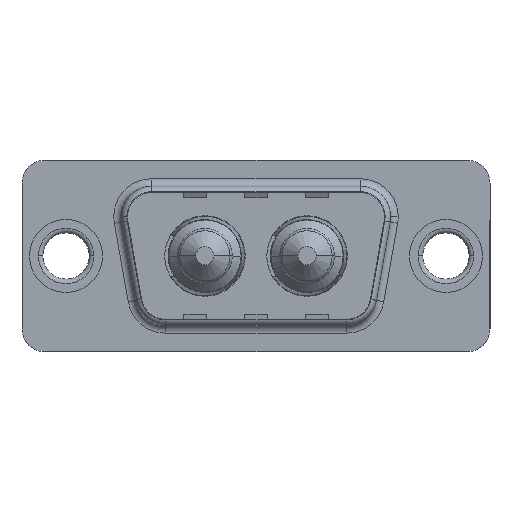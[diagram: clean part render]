
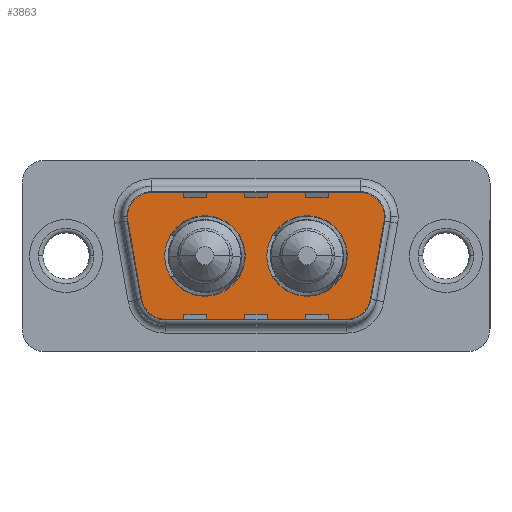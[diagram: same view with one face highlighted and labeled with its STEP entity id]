
A CAD part, top view. The second image highlights one B-rep face of the part: STEP entity #3863.
In plain terms, the highlighted planar face has unit normal (0, 0, 1).
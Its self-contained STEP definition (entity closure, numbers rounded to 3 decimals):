
#80 = VECTOR ( 'NONE', #3005, 1000. ) ;
#136 = CARTESIAN_POINT ( 'NONE',  ( 20.511, -3.247, 0. ) ) ;
#163 = EDGE_LOOP ( 'NONE', ( #2685, #4024 ) ) ;
#208 = VECTOR ( 'NONE', #8094, 1000. ) ;
#276 = CARTESIAN_POINT ( 'NONE',  ( 19.564, 2.9, 0. ) ) ;
#312 = VERTEX_POINT ( 'NONE', #4021 ) ;
#339 = ORIENTED_EDGE ( 'NONE', *, *, #7942, .F. ) ;
#349 = CARTESIAN_POINT ( 'NONE',  ( 3.466, 2.553, 0. ) ) ;
#409 = EDGE_CURVE ( 'NONE', #5698, #5153, #2336, .T. ) ;
#413 = CARTESIAN_POINT ( 'NONE',  ( 18.541, -4.9, 0. ) ) ;
#439 = FACE_OUTER_BOUND ( 'NONE', #5657, .T. ) ;
#476 = CARTESIAN_POINT ( 'NONE',  ( 18.541, -2.9, 0. ) ) ;
#579 = ORIENTED_EDGE ( 'NONE', *, *, #3668, .T. ) ;
#580 = CIRCLE ( 'NONE', #1195, 2. ) ;
#606 = DIRECTION ( 'NONE',  ( 0., 0., 1. ) ) ;
#681 = AXIS2_PLACEMENT_3D ( 'NONE', #276, #5615, #4058 ) ;
#825 = CARTESIAN_POINT ( 'NONE',  ( 9.14, 0., 0. ) ) ;
#880 = AXIS2_PLACEMENT_3D ( 'NONE', #4088, #3415, #8746 ) ;
#963 = AXIS2_PLACEMENT_3D ( 'NONE', #2575, #7895, #3344 ) ;
#983 = ORIENTED_EDGE ( 'NONE', *, *, #7571, .T. ) ;
#1108 = EDGE_LOOP ( 'NONE', ( #339, #5726 ) ) ;
#1114 = EDGE_CURVE ( 'NONE', #6469, #8653, #6492, .T. ) ;
#1126 = DIRECTION ( 'NONE',  ( 0., 0., 1. ) ) ;
#1153 = CIRCLE ( 'NONE', #963, 2.65 ) ;
#1164 = DIRECTION ( 'NONE',  ( 1., 0., 0. ) ) ;
#1195 = AXIS2_PLACEMENT_3D ( 'NONE', #5706, #1126, #6472 ) ;
#1331 = CARTESIAN_POINT ( 'NONE',  ( 6.49, 0., 0. ) ) ;
#1593 = DIRECTION ( 'NONE',  ( 1., 0., 0. ) ) ;
#2009 = ORIENTED_EDGE ( 'NONE', *, *, #2684, .T. ) ;
#2238 = FACE_BOUND ( 'NONE', #163, .T. ) ;
#2271 = EDGE_CURVE ( 'NONE', #4991, #3856, #3811, .T. ) ;
#2283 = DIRECTION ( 'NONE',  ( 0., 0., 1. ) ) ;
#2336 = CIRCLE ( 'NONE', #880, 2. ) ;
#2340 = CARTESIAN_POINT ( 'NONE',  ( 5.436, 2.9, 0. ) ) ;
#2411 = CARTESIAN_POINT ( 'NONE',  ( 15.86, 0., 0. ) ) ;
#2490 = VERTEX_POINT ( 'NONE', #349 ) ;
#2494 = CIRCLE ( 'NONE', #8648, 2. ) ;
#2575 = CARTESIAN_POINT ( 'NONE',  ( 15.86, 0., 0. ) ) ;
#2631 = VERTEX_POINT ( 'NONE', #4241 ) ;
#2684 = EDGE_CURVE ( 'NONE', #7190, #2490, #2494, .T. ) ;
#2685 = ORIENTED_EDGE ( 'NONE', *, *, #8587, .F. ) ;
#2848 = ORIENTED_EDGE ( 'NONE', *, *, #5021, .T. ) ;
#2972 = CARTESIAN_POINT ( 'NONE',  ( 6.459, -4.9, 0. ) ) ;
#3005 = DIRECTION ( 'NONE',  ( 1., 0., 0. ) ) ;
#3108 = CARTESIAN_POINT ( 'NONE',  ( 6.459, -2.9, 0. ) ) ;
#3157 = DIRECTION ( 'NONE',  ( 1., 0., 0. ) ) ;
#3291 = EDGE_CURVE ( 'NONE', #2490, #3746, #4270, .T. ) ;
#3311 = CIRCLE ( 'NONE', #7151, 2.65 ) ;
#3344 = DIRECTION ( 'NONE',  ( 1., 0., 0. ) ) ;
#3415 = DIRECTION ( 'NONE',  ( 0., 0., 1. ) ) ;
#3634 = CIRCLE ( 'NONE', #5540, 2.65 ) ;
#3668 = EDGE_CURVE ( 'NONE', #5153, #312, #7720, .T. ) ;
#3670 = VECTOR ( 'NONE', #9776, 1000. ) ;
#3722 = CARTESIAN_POINT ( 'NONE',  ( 5.436, 4.9, 0. ) ) ;
#3746 = VERTEX_POINT ( 'NONE', #8528 ) ;
#3811 = CIRCLE ( 'NONE', #681, 2. ) ;
#3856 = VERTEX_POINT ( 'NONE', #4048 ) ;
#3863 = ADVANCED_FACE ( 'NONE', ( #7821, #2238, #439 ), #4614, .T. ) ;
#3870 = DIRECTION ( 'NONE',  ( -1., 0., 0. ) ) ;
#3958 = CARTESIAN_POINT ( 'NONE',  ( 11.79, 0., 0. ) ) ;
#4021 = CARTESIAN_POINT ( 'NONE',  ( 21.534, 2.553, 0. ) ) ;
#4024 = ORIENTED_EDGE ( 'NONE', *, *, #1114, .F. ) ;
#4047 = LINE ( 'NONE', #4714, #5831 ) ;
#4048 = CARTESIAN_POINT ( 'NONE',  ( 19.564, 4.9, 0. ) ) ;
#4058 = DIRECTION ( 'NONE',  ( -1., 0., 0. ) ) ;
#4088 = CARTESIAN_POINT ( 'NONE',  ( 18.541, -2.9, 0. ) ) ;
#4241 = CARTESIAN_POINT ( 'NONE',  ( 13.21, 0., 0. ) ) ;
#4270 = LINE ( 'NONE', #9279, #208 ) ;
#4485 = AXIS2_PLACEMENT_3D ( 'NONE', #3108, #8422, #3870 ) ;
#4614 = PLANE ( 'NONE',  #8482 ) ;
#4714 = CARTESIAN_POINT ( 'NONE',  ( 5.436, 4.9, 0. ) ) ;
#4991 = VERTEX_POINT ( 'NONE', #6880 ) ;
#5021 = EDGE_CURVE ( 'NONE', #3746, #5033, #6698, .T. ) ;
#5033 = VERTEX_POINT ( 'NONE', #7675 ) ;
#5153 = VERTEX_POINT ( 'NONE', #136 ) ;
#5179 = CARTESIAN_POINT ( 'NONE',  ( 9.14, 0., 0. ) ) ;
#5280 = ORIENTED_EDGE ( 'NONE', *, *, #2271, .T. ) ;
#5540 = AXIS2_PLACEMENT_3D ( 'NONE', #825, #6160, #1593 ) ;
#5615 = DIRECTION ( 'NONE',  ( 0., 0., 1. ) ) ;
#5657 = EDGE_LOOP ( 'NONE', ( #7705, #579, #983, #5280, #7155, #2009, #7002, #2848, #6219 ) ) ;
#5698 = VERTEX_POINT ( 'NONE', #413 ) ;
#5706 = CARTESIAN_POINT ( 'NONE',  ( 19.564, 2.9, 0. ) ) ;
#5726 = ORIENTED_EDGE ( 'NONE', *, *, #6226, .F. ) ;
#5742 = DIRECTION ( 'NONE',  ( 0., 0., 1. ) ) ;
#5817 = VERTEX_POINT ( 'NONE', #7418 ) ;
#5831 = VECTOR ( 'NONE', #8497, 1000. ) ;
#5926 = LINE ( 'NONE', #2972, #80 ) ;
#5941 = DIRECTION ( 'NONE',  ( 1., 0., 0. ) ) ;
#6160 = DIRECTION ( 'NONE',  ( 0., 0., 1. ) ) ;
#6219 = ORIENTED_EDGE ( 'NONE', *, *, #6623, .T. ) ;
#6226 = EDGE_CURVE ( 'NONE', #2631, #5817, #1153, .T. ) ;
#6235 = AXIS2_PLACEMENT_3D ( 'NONE', #5179, #606, #5941 ) ;
#6469 = VERTEX_POINT ( 'NONE', #1331 ) ;
#6472 = DIRECTION ( 'NONE',  ( -1., 0., 0. ) ) ;
#6492 = CIRCLE ( 'NONE', #6235, 2.65 ) ;
#6623 = EDGE_CURVE ( 'NONE', #5033, #5698, #5926, .T. ) ;
#6642 = CARTESIAN_POINT ( 'NONE',  ( 21.534, 2.553, 0. ) ) ;
#6698 = CIRCLE ( 'NONE', #4485, 2. ) ;
#6880 = CARTESIAN_POINT ( 'NONE',  ( 21.564, 2.9, 0. ) ) ;
#7002 = ORIENTED_EDGE ( 'NONE', *, *, #3291, .T. ) ;
#7151 = AXIS2_PLACEMENT_3D ( 'NONE', #2411, #7730, #3157 ) ;
#7155 = ORIENTED_EDGE ( 'NONE', *, *, #7404, .T. ) ;
#7190 = VERTEX_POINT ( 'NONE', #3722 ) ;
#7404 = EDGE_CURVE ( 'NONE', #3856, #7190, #4047, .T. ) ;
#7418 = CARTESIAN_POINT ( 'NONE',  ( 18.51, 0., 0. ) ) ;
#7571 = EDGE_CURVE ( 'NONE', #312, #4991, #580, .T. ) ;
#7675 = CARTESIAN_POINT ( 'NONE',  ( 6.459, -4.9, 0. ) ) ;
#7705 = ORIENTED_EDGE ( 'NONE', *, *, #409, .T. ) ;
#7720 = LINE ( 'NONE', #6642, #3670 ) ;
#7730 = DIRECTION ( 'NONE',  ( 0., 0., 1. ) ) ;
#7821 = FACE_BOUND ( 'NONE', #1108, .T. ) ;
#7895 = DIRECTION ( 'NONE',  ( 0., 0., 1. ) ) ;
#7942 = EDGE_CURVE ( 'NONE', #5817, #2631, #3311, .T. ) ;
#8094 = DIRECTION ( 'NONE',  ( 0.174, -0.985, 0. ) ) ;
#8422 = DIRECTION ( 'NONE',  ( 0., 0., 1. ) ) ;
#8482 = AXIS2_PLACEMENT_3D ( 'NONE', #476, #5742, #1164 ) ;
#8497 = DIRECTION ( 'NONE',  ( -1., 0., 0. ) ) ;
#8528 = CARTESIAN_POINT ( 'NONE',  ( 4.489, -3.247, 0. ) ) ;
#8587 = EDGE_CURVE ( 'NONE', #8653, #6469, #3634, .T. ) ;
#8648 = AXIS2_PLACEMENT_3D ( 'NONE', #2340, #2283, #8772 ) ;
#8653 = VERTEX_POINT ( 'NONE', #3958 ) ;
#8746 = DIRECTION ( 'NONE',  ( 1., 0., 0. ) ) ;
#8772 = DIRECTION ( 'NONE',  ( 1., 0., 0. ) ) ;
#9279 = CARTESIAN_POINT ( 'NONE',  ( 3.466, 2.553, 0. ) ) ;
#9776 = DIRECTION ( 'NONE',  ( 0.174, 0.985, 0. ) ) ;
